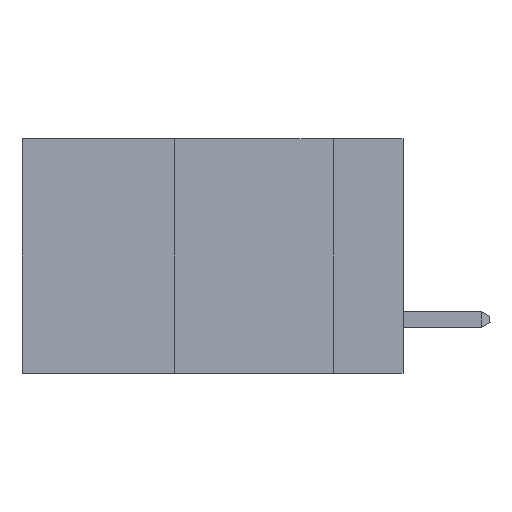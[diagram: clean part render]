
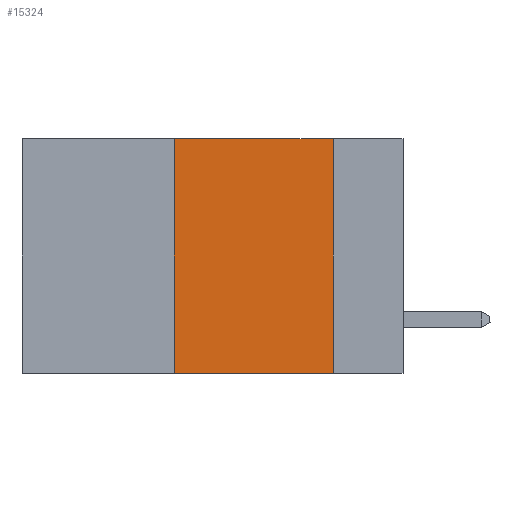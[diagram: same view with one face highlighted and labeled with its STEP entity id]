
A CAD part, left-side view. The second image highlights one B-rep face of the part: STEP entity #15324.
In plain terms, the highlighted planar face has unit normal (-1, 0, 0).
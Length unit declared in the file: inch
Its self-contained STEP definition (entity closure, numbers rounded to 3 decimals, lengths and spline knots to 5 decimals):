
#1849 = DIRECTION ( 'NONE',  ( 0., 0., 1. ) ) ;
#1903 = CARTESIAN_POINT ( 'NONE',  ( 0., 0.36, -0.37 ) ) ;
#2126 = VECTOR ( 'NONE', #21564, 39.37008 ) ;
#2802 = CARTESIAN_POINT ( 'NONE',  ( 0., 0.11, 0. ) ) ;
#2814 = ORIENTED_EDGE ( 'NONE', *, *, #32099, .F. ) ;
#4851 = LINE ( 'NONE', #22641, #9636 ) ;
#6650 = DIRECTION ( 'NONE',  ( 0., 0., -1. ) ) ;
#7186 = FACE_OUTER_BOUND ( 'NONE', #20993, .T. ) ;
#7342 = LINE ( 'NONE', #2802, #29940 ) ;
#8523 = EDGE_CURVE ( 'NONE', #22946, #32339, #4851, .T. ) ;
#9358 = VERTEX_POINT ( 'NONE', #1903 ) ;
#9478 = CARTESIAN_POINT ( 'NONE',  ( 0., 0.36, 0. ) ) ;
#9636 = VECTOR ( 'NONE', #31163, 39.37008 ) ;
#10140 = EDGE_CURVE ( 'NONE', #9358, #22946, #12183, .T. ) ;
#12183 = LINE ( 'NONE', #20429, #33510 ) ;
#12383 = CARTESIAN_POINT ( 'NONE',  ( 0., 0.6, 0. ) ) ;
#15324 = ADVANCED_FACE ( 'NONE', ( #7186 ), #20493, .F. ) ;
#17060 = AXIS2_PLACEMENT_3D ( 'NONE', #12383, #23180, #6650 ) ;
#17822 = VERTEX_POINT ( 'NONE', #23047 ) ;
#20429 = CARTESIAN_POINT ( 'NONE',  ( 0., 0.36, 0. ) ) ;
#20493 = PLANE ( 'NONE',  #17060 ) ;
#20993 = EDGE_LOOP ( 'NONE', ( #2814, #31137, #30873, #27202 ) ) ;
#21564 = DIRECTION ( 'NONE',  ( 0., -1., 0. ) ) ;
#22641 = CARTESIAN_POINT ( 'NONE',  ( 0., 0.6, 0. ) ) ;
#22946 = VERTEX_POINT ( 'NONE', #9478 ) ;
#23047 = CARTESIAN_POINT ( 'NONE',  ( 0., 0.11, -0.37 ) ) ;
#23180 = DIRECTION ( 'NONE',  ( 1., 0., 0. ) ) ;
#24281 = LINE ( 'NONE', #29106, #2126 ) ;
#27202 = ORIENTED_EDGE ( 'NONE', *, *, #33455, .T. ) ;
#29106 = CARTESIAN_POINT ( 'NONE',  ( 0., 0.6, -0.37 ) ) ;
#29940 = VECTOR ( 'NONE', #30265, 39.37008 ) ;
#30265 = DIRECTION ( 'NONE',  ( 0., 0., -1. ) ) ;
#30873 = ORIENTED_EDGE ( 'NONE', *, *, #10140, .F. ) ;
#31137 = ORIENTED_EDGE ( 'NONE', *, *, #8523, .F. ) ;
#31163 = DIRECTION ( 'NONE',  ( 0., -1., 0. ) ) ;
#31580 = CARTESIAN_POINT ( 'NONE',  ( 0., 0.11, 0. ) ) ;
#32099 = EDGE_CURVE ( 'NONE', #32339, #17822, #7342, .T. ) ;
#32339 = VERTEX_POINT ( 'NONE', #31580 ) ;
#33455 = EDGE_CURVE ( 'NONE', #9358, #17822, #24281, .T. ) ;
#33510 = VECTOR ( 'NONE', #1849, 39.37008 ) ;
